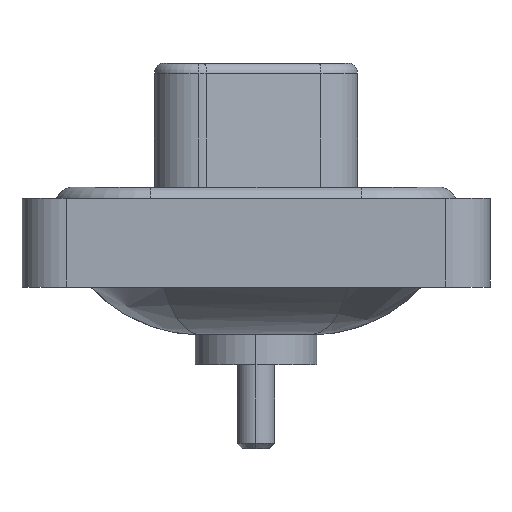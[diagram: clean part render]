
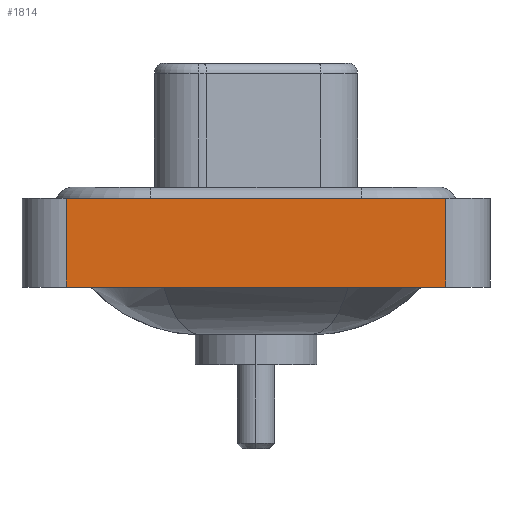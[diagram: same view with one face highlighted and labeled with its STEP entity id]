
A CAD part, left-side view. The second image highlights one B-rep face of the part: STEP entity #1814.
In plain terms, the highlighted planar face has unit normal (-1, 0, 0).
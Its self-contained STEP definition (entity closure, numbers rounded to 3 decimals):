
#236 = ORIENTED_EDGE ( 'NONE', *, *, #10769, .T. ) ;
#656 = LINE ( 'NONE', #1840, #2855 ) ;
#818 = DIRECTION ( 'NONE',  ( 0., 0., 1. ) ) ;
#1073 = LINE ( 'NONE', #3767, #4703 ) ;
#1615 = EDGE_CURVE ( 'NONE', #9818, #9769, #656, .T. ) ;
#1814 = ADVANCED_FACE ( 'NONE', ( #8679 ), #11212, .T. ) ;
#1840 = CARTESIAN_POINT ( 'NONE',  ( -7.3, -8.55, 0.4 ) ) ;
#2083 = CARTESIAN_POINT ( 'NONE',  ( -7.3, -8.55, -3.6 ) ) ;
#2364 = VERTEX_POINT ( 'NONE', #4965 ) ;
#2570 = CARTESIAN_POINT ( 'NONE',  ( -7.3, 8.55, -3.6 ) ) ;
#2792 = VECTOR ( 'NONE', #6730, 1000. ) ;
#2855 = VECTOR ( 'NONE', #6988, 1000. ) ;
#3457 = CARTESIAN_POINT ( 'NONE',  ( -7.3, -8.55, -3.6 ) ) ;
#3531 = DIRECTION ( 'NONE',  ( 0., -1., 0. ) ) ;
#3767 = CARTESIAN_POINT ( 'NONE',  ( -7.3, -8.55, -3.6 ) ) ;
#4686 = VECTOR ( 'NONE', #3531, 1000. ) ;
#4703 = VECTOR ( 'NONE', #13918, 1000. ) ;
#4965 = CARTESIAN_POINT ( 'NONE',  ( -7.3, -8.55, -3.6 ) ) ;
#5381 = LINE ( 'NONE', #15853, #2792 ) ;
#6730 = DIRECTION ( 'NONE',  ( 0., 0., 1. ) ) ;
#6988 = DIRECTION ( 'NONE',  ( 0., -1., 0. ) ) ;
#7373 = CARTESIAN_POINT ( 'NONE',  ( -7.3, 8.55, 0.4 ) ) ;
#8156 = VERTEX_POINT ( 'NONE', #2570 ) ;
#8679 = FACE_OUTER_BOUND ( 'NONE', #8900, .T. ) ;
#8900 = EDGE_LOOP ( 'NONE', ( #16052, #16245, #12292, #236 ) ) ;
#9769 = VERTEX_POINT ( 'NONE', #11960 ) ;
#9818 = VERTEX_POINT ( 'NONE', #7373 ) ;
#10769 = EDGE_CURVE ( 'NONE', #8156, #2364, #16229, .T. ) ;
#11212 = PLANE ( 'NONE',  #16619 ) ;
#11289 = EDGE_CURVE ( 'NONE', #2364, #9769, #1073, .T. ) ;
#11960 = CARTESIAN_POINT ( 'NONE',  ( -7.3, -8.55, 0.4 ) ) ;
#12292 = ORIENTED_EDGE ( 'NONE', *, *, #16022, .F. ) ;
#12389 = DIRECTION ( 'NONE',  ( -1., 0., 0. ) ) ;
#13918 = DIRECTION ( 'NONE',  ( 0., 0., 1. ) ) ;
#15853 = CARTESIAN_POINT ( 'NONE',  ( -7.3, 8.55, -3.6 ) ) ;
#16022 = EDGE_CURVE ( 'NONE', #8156, #9818, #5381, .T. ) ;
#16052 = ORIENTED_EDGE ( 'NONE', *, *, #11289, .T. ) ;
#16229 = LINE ( 'NONE', #3457, #4686 ) ;
#16245 = ORIENTED_EDGE ( 'NONE', *, *, #1615, .F. ) ;
#16619 = AXIS2_PLACEMENT_3D ( 'NONE', #2083, #12389, #818 ) ;
